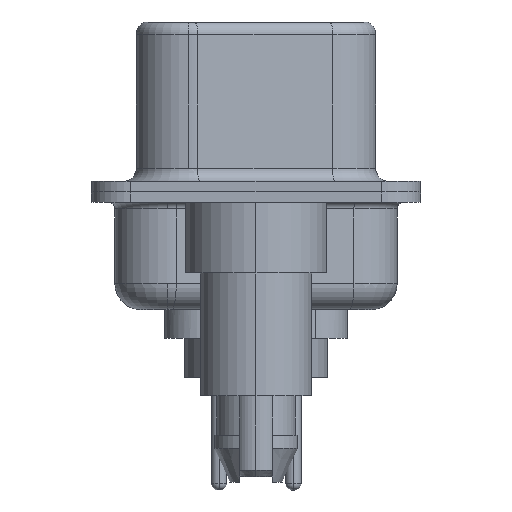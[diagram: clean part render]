
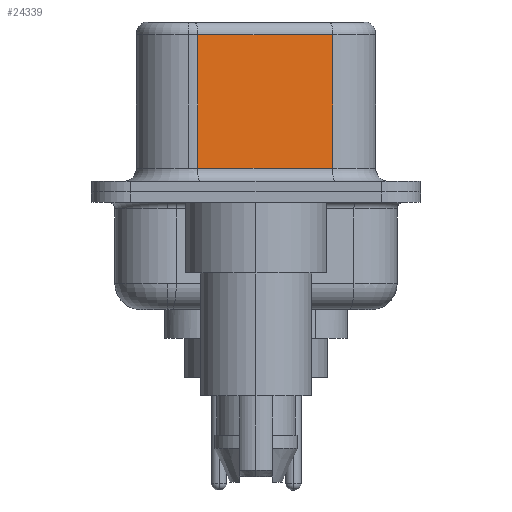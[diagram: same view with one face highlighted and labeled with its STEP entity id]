
A CAD part, left-side view. The second image highlights one B-rep face of the part: STEP entity #24339.
In plain terms, the highlighted planar face has unit normal (-0.985, -0.174, 0).
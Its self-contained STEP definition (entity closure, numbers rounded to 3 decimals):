
#918 = EDGE_CURVE ( 'NONE', #9987, #5014, #10210, .T. ) ;
#2282 = VECTOR ( 'NONE', #15496, 1000. ) ;
#2411 = DIRECTION ( 'NONE',  ( 0.985, 0.174, 0. ) ) ;
#2706 = DIRECTION ( 'NONE',  ( -0.174, 0.985, 0. ) ) ;
#5014 = VERTEX_POINT ( 'NONE', #9481 ) ;
#5559 = ORIENTED_EDGE ( 'NONE', *, *, #918, .F. ) ;
#5656 = PLANE ( 'NONE',  #12148 ) ;
#6403 = VECTOR ( 'NONE', #23135, 1000. ) ;
#7901 = VECTOR ( 'NONE', #2706, 1000. ) ;
#9024 = CARTESIAN_POINT ( 'NONE',  ( 4.585, -2.927, 0.9 ) ) ;
#9481 = CARTESIAN_POINT ( 'NONE',  ( 4.585, -2.927, 0.9 ) ) ;
#9708 = ORIENTED_EDGE ( 'NONE', *, *, #20653, .T. ) ;
#9987 = VERTEX_POINT ( 'NONE', #13656 ) ;
#10210 = LINE ( 'NONE', #19545, #6403 ) ;
#10890 = VERTEX_POINT ( 'NONE', #23837 ) ;
#11500 = EDGE_LOOP ( 'NONE', ( #5559, #22978, #9708, #16435 ) ) ;
#11607 = DIRECTION ( 'NONE',  ( -0.174, 0.985, 0. ) ) ;
#12148 = AXIS2_PLACEMENT_3D ( 'NONE', #22837, #2411, #11607 ) ;
#13407 = FACE_OUTER_BOUND ( 'NONE', #11500, .T. ) ;
#13592 = VECTOR ( 'NONE', #18566, 1000. ) ;
#13656 = CARTESIAN_POINT ( 'NONE',  ( 4.585, -2.927, 6.02 ) ) ;
#13856 = LINE ( 'NONE', #9024, #13592 ) ;
#13919 = EDGE_CURVE ( 'NONE', #9987, #19697, #22961, .T. ) ;
#15496 = DIRECTION ( 'NONE',  ( 0., 0., -1. ) ) ;
#16435 = ORIENTED_EDGE ( 'NONE', *, *, #19784, .T. ) ;
#17094 = LINE ( 'NONE', #19266, #2282 ) ;
#18179 = CARTESIAN_POINT ( 'NONE',  ( 3.675, 2.233, 6.02 ) ) ;
#18566 = DIRECTION ( 'NONE',  ( 0.174, -0.985, 0. ) ) ;
#19266 = CARTESIAN_POINT ( 'NONE',  ( 3.675, 2.233, 6.52 ) ) ;
#19474 = CARTESIAN_POINT ( 'NONE',  ( 4.585, -2.927, 6.02 ) ) ;
#19545 = CARTESIAN_POINT ( 'NONE',  ( 4.585, -2.927, 6.52 ) ) ;
#19697 = VERTEX_POINT ( 'NONE', #18179 ) ;
#19784 = EDGE_CURVE ( 'NONE', #10890, #5014, #13856, .T. ) ;
#20653 = EDGE_CURVE ( 'NONE', #19697, #10890, #17094, .T. ) ;
#22837 = CARTESIAN_POINT ( 'NONE',  ( 4.585, -2.927, 6.52 ) ) ;
#22961 = LINE ( 'NONE', #19474, #7901 ) ;
#22978 = ORIENTED_EDGE ( 'NONE', *, *, #13919, .T. ) ;
#23135 = DIRECTION ( 'NONE',  ( 0., 0., -1. ) ) ;
#23837 = CARTESIAN_POINT ( 'NONE',  ( 3.675, 2.233, 0.9 ) ) ;
#24339 = ADVANCED_FACE ( 'NONE', ( #13407 ), #5656, .F. ) ;
